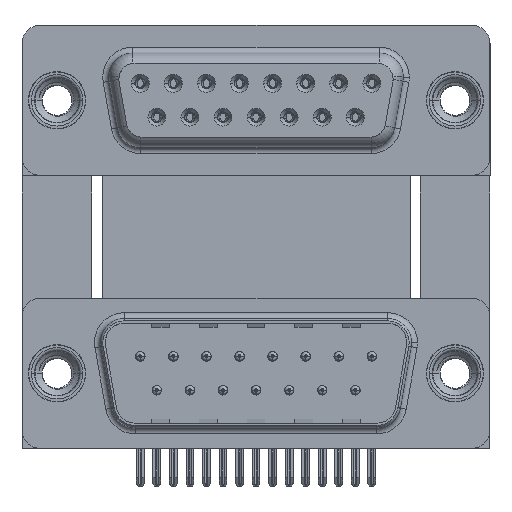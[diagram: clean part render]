
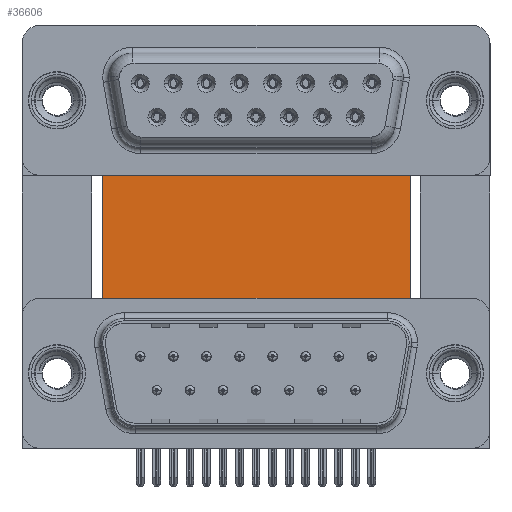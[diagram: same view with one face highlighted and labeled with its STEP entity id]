
A CAD part, top view. The second image highlights one B-rep face of the part: STEP entity #36606.
In plain terms, the highlighted planar face has unit normal (0, 0, 1).
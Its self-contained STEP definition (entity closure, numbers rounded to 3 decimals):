
#1849 = CARTESIAN_POINT ( 'NONE',  ( 3.79, -3.735, -12. ) ) ;
#4290 = VECTOR ( 'NONE', #33002, 1000. ) ;
#5632 = DIRECTION ( 'NONE',  ( 0., -1., 0. ) ) ;
#6086 = ORIENTED_EDGE ( 'NONE', *, *, #25404, .T. ) ;
#9447 = FACE_OUTER_BOUND ( 'NONE', #23239, .T. ) ;
#10381 = AXIS2_PLACEMENT_3D ( 'NONE', #23225, #12559, #36825 ) ;
#10699 = CARTESIAN_POINT ( 'NONE',  ( 29.58, 16.585, -12. ) ) ;
#12559 = DIRECTION ( 'NONE',  ( 0., 0., -1. ) ) ;
#13572 = VERTEX_POINT ( 'NONE', #10699 ) ;
#16082 = CARTESIAN_POINT ( 'NONE',  ( 3.79, 16.585, -12. ) ) ;
#17300 = LINE ( 'NONE', #37560, #38026 ) ;
#19315 = CARTESIAN_POINT ( 'NONE',  ( 3.79, -3.735, -12. ) ) ;
#19432 = LINE ( 'NONE', #1849, #4290 ) ;
#20396 = CARTESIAN_POINT ( 'NONE',  ( 3.79, 16.585, -12. ) ) ;
#23212 = VERTEX_POINT ( 'NONE', #19315 ) ;
#23225 = CARTESIAN_POINT ( 'NONE',  ( 3.79, 16.585, -12. ) ) ;
#23232 = VECTOR ( 'NONE', #29777, 1000. ) ;
#23239 = EDGE_LOOP ( 'NONE', ( #26339, #36566, #27148, #6086 ) ) ;
#23399 = EDGE_CURVE ( 'NONE', #38337, #13572, #43592, .T. ) ;
#25404 = EDGE_CURVE ( 'NONE', #38337, #23212, #39486, .T. ) ;
#25927 = PLANE ( 'NONE',  #10381 ) ;
#26339 = ORIENTED_EDGE ( 'NONE', *, *, #27178, .T. ) ;
#26376 = VERTEX_POINT ( 'NONE', #36896 ) ;
#27148 = ORIENTED_EDGE ( 'NONE', *, *, #23399, .F. ) ;
#27178 = EDGE_CURVE ( 'NONE', #23212, #26376, #19432, .T. ) ;
#29777 = DIRECTION ( 'NONE',  ( 1., 0., 0. ) ) ;
#33002 = DIRECTION ( 'NONE',  ( 1., 0., 0. ) ) ;
#34355 = EDGE_CURVE ( 'NONE', #13572, #26376, #17300, .T. ) ;
#34778 = VECTOR ( 'NONE', #5632, 1000. ) ;
#36141 = CARTESIAN_POINT ( 'NONE',  ( 3.79, 16.585, -12. ) ) ;
#36566 = ORIENTED_EDGE ( 'NONE', *, *, #34355, .F. ) ;
#36606 = ADVANCED_FACE ( 'NONE', ( #9447 ), #25927, .F. ) ;
#36825 = DIRECTION ( 'NONE',  ( -1., 0., 0. ) ) ;
#36896 = CARTESIAN_POINT ( 'NONE',  ( 29.58, -3.735, -12. ) ) ;
#37338 = DIRECTION ( 'NONE',  ( 0., -1., 0. ) ) ;
#37560 = CARTESIAN_POINT ( 'NONE',  ( 29.58, 16.585, -12. ) ) ;
#38026 = VECTOR ( 'NONE', #37338, 1000. ) ;
#38337 = VERTEX_POINT ( 'NONE', #16082 ) ;
#39486 = LINE ( 'NONE', #36141, #34778 ) ;
#43592 = LINE ( 'NONE', #20396, #23232 ) ;
